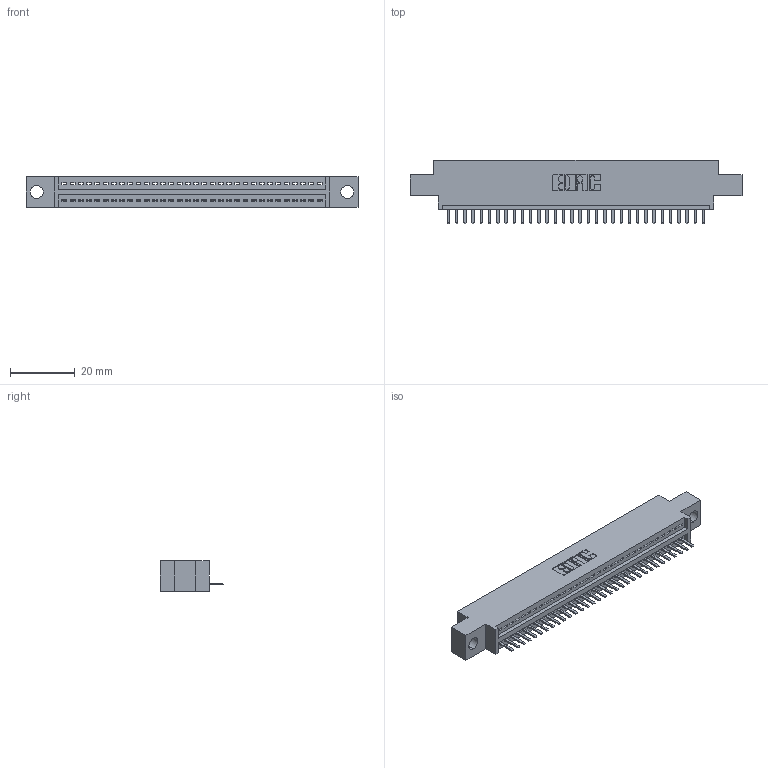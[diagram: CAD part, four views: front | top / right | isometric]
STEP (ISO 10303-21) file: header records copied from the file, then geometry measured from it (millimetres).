
FILE_DESCRIPTION (( 'STEP AP203' ), '1' );
FILE_NAME ('395-032-520-604.STEP', '2018-11-12T17:52:52', ( '' ), ( '' ), 'SwSTEP 2.0', 'SolidWorks 2016', '' );
FILE_SCHEMA (( 'CONFIG_CONTROL_DESIGN' ));
Length unit declared in the file: inch
Products named in the file (3): 345 Part_0.170 Offset - 0.156 Dia-TH; 395-032-520-604; 345-292-001_345-293-120
Assembly tree (33 placements, depth 2):
  395-032-520-604
    345 Part_0.170 Offset - 0.156 Dia-TH
    345-292-001_345-293-120  x32
Bounding box: 102.49 x 19.68 x 9.4 mm (x, y, z)
Volume: 9359.3 mm3; surface area: 11935.9 mm2
Topology: 33 solids, 33 shells, 2114 faces, 6241 edges, 4074 vertices
Faces by surface type: plane 1428, cylinder 686
Entity records: 25679 total; most frequent: CARTESIAN_POINT 4468, ORIENTED_EDGE 4422, DIRECTION 3903, EDGE_CURVE 2211, VECTOR 1947, LINE 1947, VERTEX_POINT 1470, AXIS2_PLACEMENT_3D 978
